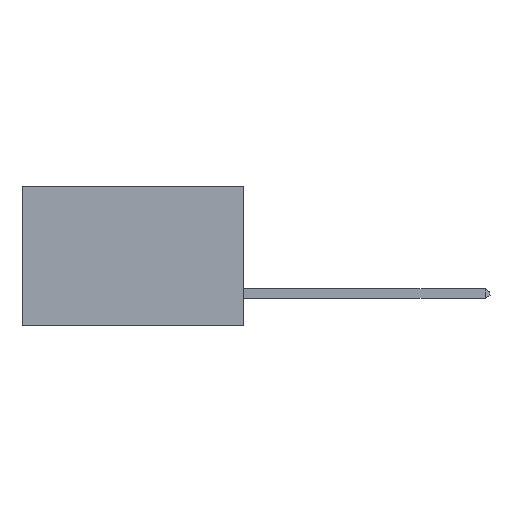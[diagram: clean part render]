
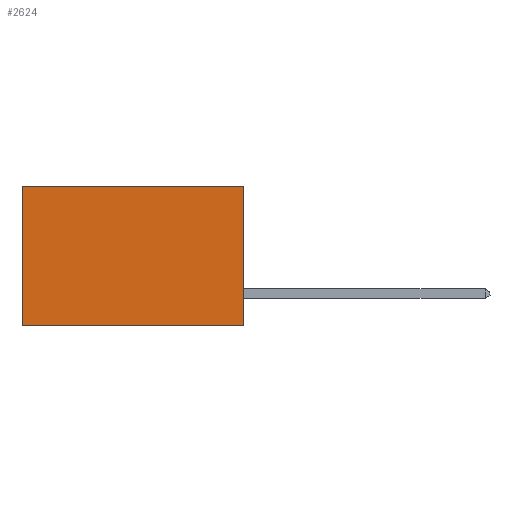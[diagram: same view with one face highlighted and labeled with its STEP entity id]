
A CAD part, left-side view. The second image highlights one B-rep face of the part: STEP entity #2624.
In plain terms, the highlighted planar face has unit normal (-1, 0, 0).
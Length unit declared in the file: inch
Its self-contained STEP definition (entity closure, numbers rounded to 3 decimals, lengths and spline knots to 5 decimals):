
#126 = VECTOR ( 'NONE', #13181, 39.37008 ) ;
#896 = LINE ( 'NONE', #1354, #11833 ) ;
#1147 = DIRECTION ( 'NONE',  ( 0., 0., -1. ) ) ;
#1354 = CARTESIAN_POINT ( 'NONE',  ( 0.277, 0.59, -0.37 ) ) ;
#1419 = ORIENTED_EDGE ( 'NONE', *, *, #7111, .T. ) ;
#1904 = VERTEX_POINT ( 'NONE', #11736 ) ;
#2166 = EDGE_CURVE ( 'NONE', #11681, #6424, #11653, .T. ) ;
#2242 = DIRECTION ( 'NONE',  ( 0., 1., 0. ) ) ;
#2624 = ADVANCED_FACE ( 'NONE', ( #5792 ), #7160, .F. ) ;
#2735 = CARTESIAN_POINT ( 'NONE',  ( 0.277, 0., 0. ) ) ;
#2952 = CARTESIAN_POINT ( 'NONE',  ( 0.277, 0., 0. ) ) ;
#3265 = DIRECTION ( 'NONE',  ( 0., 1., 0. ) ) ;
#3573 = EDGE_CURVE ( 'NONE', #7412, #1904, #8877, .T. ) ;
#4382 = LINE ( 'NONE', #14224, #126 ) ;
#5065 = AXIS2_PLACEMENT_3D ( 'NONE', #8000, #6886, #6872 ) ;
#5446 = VECTOR ( 'NONE', #3265, 39.37008 ) ;
#5502 = CARTESIAN_POINT ( 'NONE',  ( 0.277, 0., -0.37 ) ) ;
#5792 = FACE_OUTER_BOUND ( 'NONE', #10075, .T. ) ;
#6424 = VERTEX_POINT ( 'NONE', #8985 ) ;
#6872 = DIRECTION ( 'NONE',  ( 0., 0., -1. ) ) ;
#6886 = DIRECTION ( 'NONE',  ( 1., 0., 0. ) ) ;
#7111 = EDGE_CURVE ( 'NONE', #1904, #6424, #896, .T. ) ;
#7160 = PLANE ( 'NONE',  #5065 ) ;
#7412 = VERTEX_POINT ( 'NONE', #2735 ) ;
#8000 = CARTESIAN_POINT ( 'NONE',  ( 0.277, 0., -0.37 ) ) ;
#8535 = VECTOR ( 'NONE', #2242, 39.37008 ) ;
#8877 = LINE ( 'NONE', #2952, #8535 ) ;
#8985 = CARTESIAN_POINT ( 'NONE',  ( 0.277, 0.59, -0.37 ) ) ;
#10075 = EDGE_LOOP ( 'NONE', ( #1419, #12872, #12921, #12310 ) ) ;
#10153 = CARTESIAN_POINT ( 'NONE',  ( 0.277, 0., -0.37 ) ) ;
#11653 = LINE ( 'NONE', #10153, #5446 ) ;
#11681 = VERTEX_POINT ( 'NONE', #5502 ) ;
#11736 = CARTESIAN_POINT ( 'NONE',  ( 0.277, 0.59, 0. ) ) ;
#11833 = VECTOR ( 'NONE', #1147, 39.37008 ) ;
#12310 = ORIENTED_EDGE ( 'NONE', *, *, #3573, .T. ) ;
#12872 = ORIENTED_EDGE ( 'NONE', *, *, #2166, .F. ) ;
#12921 = ORIENTED_EDGE ( 'NONE', *, *, #14340, .F. ) ;
#13181 = DIRECTION ( 'NONE',  ( 0., 0., -1. ) ) ;
#14224 = CARTESIAN_POINT ( 'NONE',  ( 0.277, 0., -0.37 ) ) ;
#14340 = EDGE_CURVE ( 'NONE', #7412, #11681, #4382, .T. ) ;
